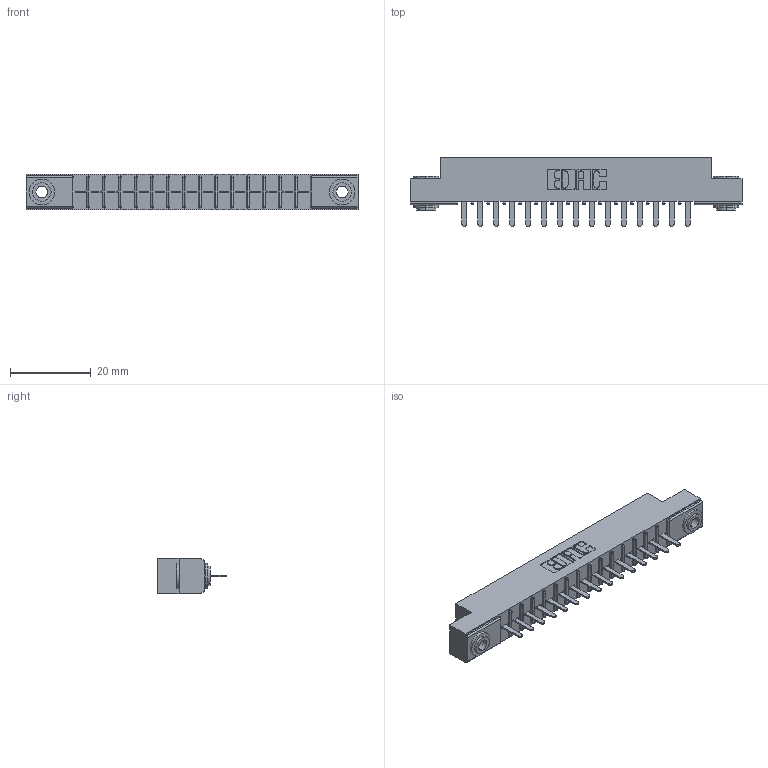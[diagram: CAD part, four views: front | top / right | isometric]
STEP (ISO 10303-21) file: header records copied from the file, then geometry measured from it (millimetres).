
FILE_DESCRIPTION (( 'STEP AP203' ), '1' );
FILE_NAME ('356-015-520-103.STEP', '2018-08-01T19:10:30', ( '' ), ( '' ), 'SwSTEP 2.0', 'SolidWorks 2016', '' );
FILE_SCHEMA (( 'CONFIG_CONTROL_DESIGN' ));
Length unit declared in the file: inch
Products named in the file (4): 306 Part_.156 Dia; 306-290-001_120; 345-250-002_345-250-002-102; 356-015-520-103
Assembly tree (18 placements, depth 2):
  356-015-520-103
    306 Part_.156 Dia
    306-290-001_120  x15
    345-250-002_345-250-002-102  x2
Bounding box: 82.45 x 17.12 x 8.71 mm (x, y, z)
Volume: 5607.4 mm3; surface area: 8333.7 mm2
Topology: 18 solids, 18 shells, 1218 faces, 3383 edges, 2170 vertices
Faces by surface type: plane 797, cylinder 353, sphere 60, cone 8
Entity records: 18507 total; most frequent: CARTESIAN_POINT 3081, DIRECTION 3055, ORIENTED_EDGE 3042, EDGE_CURVE 1521, LINE 1167, VECTOR 1167, VERTEX_POINT 970, AXIS2_PLACEMENT_3D 944
